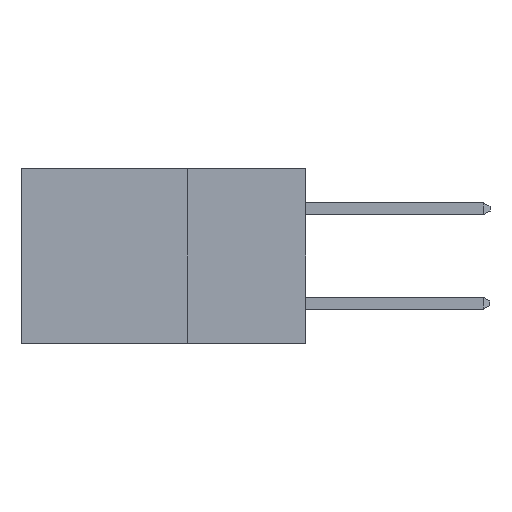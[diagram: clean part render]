
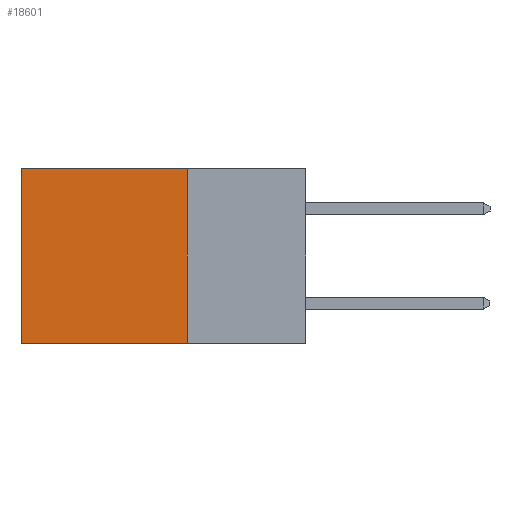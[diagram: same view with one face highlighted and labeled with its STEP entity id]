
A CAD part, left-side view. The second image highlights one B-rep face of the part: STEP entity #18601.
In plain terms, the highlighted planar face has unit normal (-1, 0, 0).
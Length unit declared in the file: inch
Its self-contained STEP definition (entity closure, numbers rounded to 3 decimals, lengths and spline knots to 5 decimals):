
#903 = CARTESIAN_POINT ( 'NONE',  ( 0.298, 0.25, 0. ) ) ;
#1776 = AXIS2_PLACEMENT_3D ( 'NONE', #903, #15504, #3013 ) ;
#2035 = FACE_OUTER_BOUND ( 'NONE', #25486, .T. ) ;
#2971 = VERTEX_POINT ( 'NONE', #5263 ) ;
#3013 = DIRECTION ( 'NONE',  ( 0., 0., -1. ) ) ;
#4423 = LINE ( 'NONE', #7972, #20325 ) ;
#4577 = VECTOR ( 'NONE', #24739, 39.37008 ) ;
#4840 = ORIENTED_EDGE ( 'NONE', *, *, #19789, .F. ) ;
#5125 = ORIENTED_EDGE ( 'NONE', *, *, #14544, .F. ) ;
#5263 = CARTESIAN_POINT ( 'NONE',  ( 0.298, 0.6, 0. ) ) ;
#5444 = CARTESIAN_POINT ( 'NONE',  ( 0.298, 0.25, 0. ) ) ;
#6566 = VECTOR ( 'NONE', #6780, 39.37008 ) ;
#6780 = DIRECTION ( 'NONE',  ( 0., 1., 0. ) ) ;
#7556 = DIRECTION ( 'NONE',  ( 0., 0., -1. ) ) ;
#7685 = VERTEX_POINT ( 'NONE', #16985 ) ;
#7972 = CARTESIAN_POINT ( 'NONE',  ( 0.298, 0.6, 0. ) ) ;
#8065 = DIRECTION ( 'NONE',  ( 0., 0., -1. ) ) ;
#8277 = CARTESIAN_POINT ( 'NONE',  ( 0.298, 0.25, -0.37 ) ) ;
#8847 = LINE ( 'NONE', #5444, #24614 ) ;
#11697 = EDGE_CURVE ( 'NONE', #2971, #7685, #4423, .T. ) ;
#13106 = CARTESIAN_POINT ( 'NONE',  ( 0.298, 0.25, 0. ) ) ;
#14544 = EDGE_CURVE ( 'NONE', #17910, #23292, #8847, .T. ) ;
#15504 = DIRECTION ( 'NONE',  ( 1., 0., 0. ) ) ;
#16912 = ORIENTED_EDGE ( 'NONE', *, *, #11697, .T. ) ;
#16985 = CARTESIAN_POINT ( 'NONE',  ( 0.298, 0.6, -0.37 ) ) ;
#17369 = ORIENTED_EDGE ( 'NONE', *, *, #22025, .T. ) ;
#17910 = VERTEX_POINT ( 'NONE', #13106 ) ;
#18259 = LINE ( 'NONE', #19275, #6566 ) ;
#18601 = ADVANCED_FACE ( 'NONE', ( #2035 ), #21612, .F. ) ;
#18812 = CARTESIAN_POINT ( 'NONE',  ( 0.298, 0.25, -0.37 ) ) ;
#19275 = CARTESIAN_POINT ( 'NONE',  ( 0.298, 0.25, 0. ) ) ;
#19789 = EDGE_CURVE ( 'NONE', #23292, #7685, #26515, .T. ) ;
#20325 = VECTOR ( 'NONE', #8065, 39.37008 ) ;
#21612 = PLANE ( 'NONE',  #1776 ) ;
#22025 = EDGE_CURVE ( 'NONE', #17910, #2971, #18259, .T. ) ;
#23292 = VERTEX_POINT ( 'NONE', #18812 ) ;
#24614 = VECTOR ( 'NONE', #7556, 39.37008 ) ;
#24739 = DIRECTION ( 'NONE',  ( 0., 1., 0. ) ) ;
#25486 = EDGE_LOOP ( 'NONE', ( #16912, #4840, #5125, #17369 ) ) ;
#26515 = LINE ( 'NONE', #8277, #4577 ) ;
